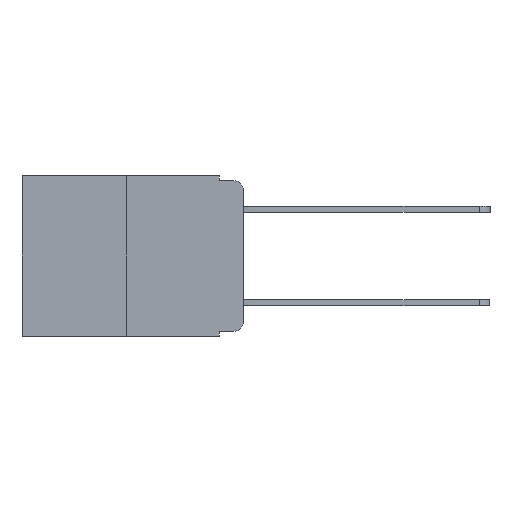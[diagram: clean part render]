
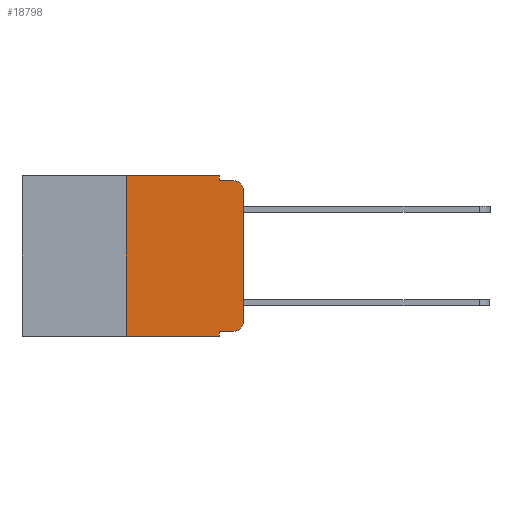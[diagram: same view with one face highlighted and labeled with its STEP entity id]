
A CAD part, left-side view. The second image highlights one B-rep face of the part: STEP entity #18798.
In plain terms, the highlighted planar face has unit normal (-1, 0, 0).
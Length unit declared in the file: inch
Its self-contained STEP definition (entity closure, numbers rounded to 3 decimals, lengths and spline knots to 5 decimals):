
#203 = VECTOR ( 'NONE', #12149, 39.37008 ) ;
#325 = DIRECTION ( 'NONE',  ( 0., 0., -1. ) ) ;
#646 = CARTESIAN_POINT ( 'NONE',  ( 0., 0.473, 0. ) ) ;
#988 = AXIS2_PLACEMENT_3D ( 'NONE', #6436, #2362, #2097 ) ;
#1034 = CARTESIAN_POINT ( 'NONE',  ( 0., 0.051, 0. ) ) ;
#1228 = DIRECTION ( 'NONE',  ( 0., 0., 1. ) ) ;
#1588 = CARTESIAN_POINT ( 'NONE',  ( 0., 0.25, -0.343 ) ) ;
#1767 = VERTEX_POINT ( 'NONE', #15662 ) ;
#1958 = EDGE_CURVE ( 'NONE', #12525, #6592, #11682, .T. ) ;
#2097 = DIRECTION ( 'NONE',  ( 0., 0., -1. ) ) ;
#2117 = ORIENTED_EDGE ( 'NONE', *, *, #9069, .F. ) ;
#2122 = CARTESIAN_POINT ( 'NONE',  ( 0., 0.02, -0.333 ) ) ;
#2267 = LINE ( 'NONE', #22678, #20523 ) ;
#2362 = DIRECTION ( 'NONE',  ( -1., 0., 0. ) ) ;
#2397 = EDGE_CURVE ( 'NONE', #16406, #4865, #8058, .T. ) ;
#2713 = CARTESIAN_POINT ( 'NONE',  ( 0., 0.051, -0.343 ) ) ;
#2938 = AXIS2_PLACEMENT_3D ( 'NONE', #16261, #10520, #325 ) ;
#2993 = LINE ( 'NONE', #20468, #11939 ) ;
#4737 = ORIENTED_EDGE ( 'NONE', *, *, #10582, .T. ) ;
#4865 = VERTEX_POINT ( 'NONE', #18356 ) ;
#5115 = DIRECTION ( 'NONE',  ( 0., 0., -1. ) ) ;
#5196 = DIRECTION ( 'NONE',  ( 0., -1., 0. ) ) ;
#5653 = ORIENTED_EDGE ( 'NONE', *, *, #18439, .T. ) ;
#6056 = PLANE ( 'NONE',  #14208 ) ;
#6383 = DIRECTION ( 'NONE',  ( 0., 0., 1. ) ) ;
#6436 = CARTESIAN_POINT ( 'NONE',  ( 0., 0.02, -0.03 ) ) ;
#6498 = VERTEX_POINT ( 'NONE', #2713 ) ;
#6592 = VERTEX_POINT ( 'NONE', #17244 ) ;
#6880 = VECTOR ( 'NONE', #14474, 39.37008 ) ;
#6882 = CARTESIAN_POINT ( 'NONE',  ( 0., 0.051, 0. ) ) ;
#7717 = ORIENTED_EDGE ( 'NONE', *, *, #12853, .F. ) ;
#7853 = DIRECTION ( 'NONE',  ( 1., 0., 0. ) ) ;
#8058 = CIRCLE ( 'NONE', #2938, 0.02 ) ;
#8213 = EDGE_CURVE ( 'NONE', #1767, #6498, #9764, .T. ) ;
#8264 = ORIENTED_EDGE ( 'NONE', *, *, #10077, .T. ) ;
#9022 = ORIENTED_EDGE ( 'NONE', *, *, #1958, .T. ) ;
#9069 = EDGE_CURVE ( 'NONE', #13358, #6592, #11641, .T. ) ;
#9364 = LINE ( 'NONE', #22314, #18146 ) ;
#9764 = LINE ( 'NONE', #6882, #16899 ) ;
#9886 = VERTEX_POINT ( 'NONE', #1034 ) ;
#9887 = VECTOR ( 'NONE', #15930, 39.37008 ) ;
#10077 = EDGE_CURVE ( 'NONE', #1767, #16406, #15124, .T. ) ;
#10516 = CARTESIAN_POINT ( 'NONE',  ( 0., 0.051, -0.333 ) ) ;
#10520 = DIRECTION ( 'NONE',  ( -1., 0., 0. ) ) ;
#10582 = EDGE_CURVE ( 'NONE', #4865, #12525, #9364, .T. ) ;
#10608 = ORIENTED_EDGE ( 'NONE', *, *, #8213, .F. ) ;
#11485 = EDGE_LOOP ( 'NONE', ( #4737, #9022, #2117, #15015, #7717, #13372, #5653, #10608, #8264, #18319 ) ) ;
#11641 = LINE ( 'NONE', #19732, #6880 ) ;
#11682 = CIRCLE ( 'NONE', #988, 0.02 ) ;
#11939 = VECTOR ( 'NONE', #6383, 39.37008 ) ;
#12149 = DIRECTION ( 'NONE',  ( 0., -1., 0. ) ) ;
#12216 = VERTEX_POINT ( 'NONE', #1588 ) ;
#12525 = VERTEX_POINT ( 'NONE', #18544 ) ;
#12853 = EDGE_CURVE ( 'NONE', #19828, #9886, #14499, .T. ) ;
#13358 = VERTEX_POINT ( 'NONE', #22459 ) ;
#13372 = ORIENTED_EDGE ( 'NONE', *, *, #18313, .F. ) ;
#13414 = EDGE_CURVE ( 'NONE', #9886, #13358, #2267, .T. ) ;
#14208 = AXIS2_PLACEMENT_3D ( 'NONE', #646, #7853, #20153 ) ;
#14474 = DIRECTION ( 'NONE',  ( 0., -1., 0. ) ) ;
#14499 = LINE ( 'NONE', #16010, #9887 ) ;
#15015 = ORIENTED_EDGE ( 'NONE', *, *, #13414, .F. ) ;
#15059 = CARTESIAN_POINT ( 'NONE',  ( 0., 0.25, 0. ) ) ;
#15124 = LINE ( 'NONE', #10516, #19279 ) ;
#15662 = CARTESIAN_POINT ( 'NONE',  ( 0., 0.051, -0.333 ) ) ;
#15930 = DIRECTION ( 'NONE',  ( 0., -1., 0. ) ) ;
#16010 = CARTESIAN_POINT ( 'NONE',  ( 0., 0.473, 0. ) ) ;
#16261 = CARTESIAN_POINT ( 'NONE',  ( 0., 0.02, -0.313 ) ) ;
#16406 = VERTEX_POINT ( 'NONE', #2122 ) ;
#16573 = FACE_OUTER_BOUND ( 'NONE', #11485, .T. ) ;
#16899 = VECTOR ( 'NONE', #5115, 39.37008 ) ;
#17244 = CARTESIAN_POINT ( 'NONE',  ( 0., 0.02, -0.01 ) ) ;
#17631 = DIRECTION ( 'NONE',  ( 0., 0., -1. ) ) ;
#18146 = VECTOR ( 'NONE', #1228, 39.37008 ) ;
#18313 = EDGE_CURVE ( 'NONE', #12216, #19828, #2993, .T. ) ;
#18319 = ORIENTED_EDGE ( 'NONE', *, *, #2397, .T. ) ;
#18356 = CARTESIAN_POINT ( 'NONE',  ( 0., 0., -0.313 ) ) ;
#18439 = EDGE_CURVE ( 'NONE', #12216, #6498, #18489, .T. ) ;
#18489 = LINE ( 'NONE', #22505, #203 ) ;
#18544 = CARTESIAN_POINT ( 'NONE',  ( 0., 0., -0.03 ) ) ;
#18798 = ADVANCED_FACE ( 'NONE', ( #16573 ), #6056, .F. ) ;
#19279 = VECTOR ( 'NONE', #5196, 39.37008 ) ;
#19732 = CARTESIAN_POINT ( 'NONE',  ( 0., 0.051, -0.01 ) ) ;
#19828 = VERTEX_POINT ( 'NONE', #15059 ) ;
#20153 = DIRECTION ( 'NONE',  ( 0., 0., -1. ) ) ;
#20468 = CARTESIAN_POINT ( 'NONE',  ( 0., 0.25, 0. ) ) ;
#20523 = VECTOR ( 'NONE', #17631, 39.37008 ) ;
#22314 = CARTESIAN_POINT ( 'NONE',  ( 0., 0., 0. ) ) ;
#22459 = CARTESIAN_POINT ( 'NONE',  ( 0., 0.051, -0.01 ) ) ;
#22505 = CARTESIAN_POINT ( 'NONE',  ( 0., 0.473, -0.343 ) ) ;
#22678 = CARTESIAN_POINT ( 'NONE',  ( 0., 0.051, 0. ) ) ;
